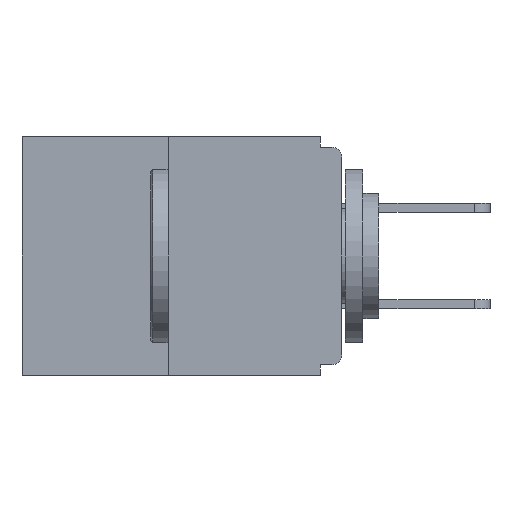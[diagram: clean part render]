
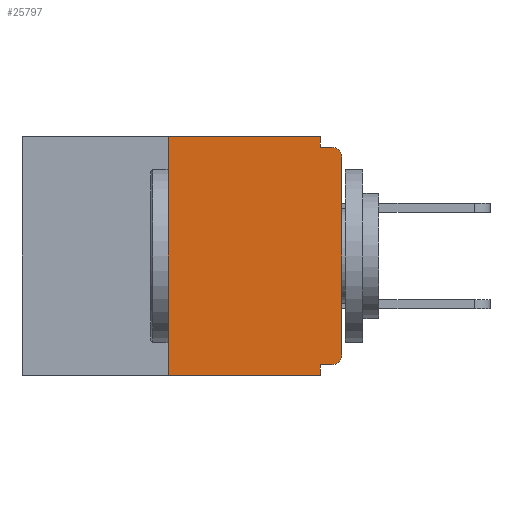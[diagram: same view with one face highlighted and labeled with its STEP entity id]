
A CAD part, left-side view. The second image highlights one B-rep face of the part: STEP entity #25797.
In plain terms, the highlighted planar face has unit normal (-1, 0, 0).
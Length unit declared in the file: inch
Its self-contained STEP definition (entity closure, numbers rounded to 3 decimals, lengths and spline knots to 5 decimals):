
#19 = VECTOR ( 'NONE', #25999, 39.37008 ) ;
#144 = DIRECTION ( 'NONE',  ( 0., -1., 0. ) ) ;
#310 = VERTEX_POINT ( 'NONE', #5713 ) ;
#333 = EDGE_CURVE ( 'NONE', #24764, #22253, #2585, .T. ) ;
#414 = DIRECTION ( 'NONE',  ( 0., -1., 0. ) ) ;
#470 = DIRECTION ( 'NONE',  ( 0., 0., -1. ) ) ;
#1014 = DIRECTION ( 'NONE',  ( 0., 0., -1. ) ) ;
#1620 = VECTOR ( 'NONE', #14173, 39.37008 ) ;
#2585 = LINE ( 'NONE', #15655, #19 ) ;
#3211 = VECTOR ( 'NONE', #24478, 39.37008 ) ;
#3716 = CARTESIAN_POINT ( 'NONE',  ( 0., 0.031, 0. ) ) ;
#3780 = EDGE_CURVE ( 'NONE', #19510, #6111, #23849, .T. ) ;
#3953 = ORIENTED_EDGE ( 'NONE', *, *, #10711, .T. ) ;
#4351 = LINE ( 'NONE', #12696, #9069 ) ;
#4534 = PLANE ( 'NONE',  #5822 ) ;
#4658 = ORIENTED_EDGE ( 'NONE', *, *, #8593, .F. ) ;
#4842 = VECTOR ( 'NONE', #414, 39.37008 ) ;
#5281 = DIRECTION ( 'NONE',  ( 0., 0., -1. ) ) ;
#5429 = ORIENTED_EDGE ( 'NONE', *, *, #17405, .F. ) ;
#5528 = CARTESIAN_POINT ( 'NONE',  ( 0., 0.25, 0. ) ) ;
#5553 = LINE ( 'NONE', #20204, #12527 ) ;
#5713 = CARTESIAN_POINT ( 'NONE',  ( 0., 0.25, -0.343 ) ) ;
#5822 = AXIS2_PLACEMENT_3D ( 'NONE', #22759, #24715, #470 ) ;
#6111 = VERTEX_POINT ( 'NONE', #15145 ) ;
#6182 = ORIENTED_EDGE ( 'NONE', *, *, #19927, .F. ) ;
#6338 = EDGE_CURVE ( 'NONE', #13359, #7127, #8822, .T. ) ;
#6804 = ORIENTED_EDGE ( 'NONE', *, *, #23769, .F. ) ;
#7127 = VERTEX_POINT ( 'NONE', #23891 ) ;
#7247 = EDGE_CURVE ( 'NONE', #21925, #22702, #4351, .T. ) ;
#7382 = DIRECTION ( 'NONE',  ( 0., 0., 1. ) ) ;
#8100 = EDGE_CURVE ( 'NONE', #6111, #13359, #17264, .T. ) ;
#8593 = EDGE_CURVE ( 'NONE', #22253, #7127, #5553, .T. ) ;
#8822 = CIRCLE ( 'NONE', #13128, 0.015 ) ;
#8937 = DIRECTION ( 'NONE',  ( -1., 0., 0. ) ) ;
#9069 = VECTOR ( 'NONE', #12786, 39.37008 ) ;
#9969 = VECTOR ( 'NONE', #21631, 39.37008 ) ;
#10627 = CARTESIAN_POINT ( 'NONE',  ( 0., 0.46, -0.343 ) ) ;
#10711 = EDGE_CURVE ( 'NONE', #310, #22702, #15845, .T. ) ;
#10890 = CARTESIAN_POINT ( 'NONE',  ( 0., 0.015, -0.03 ) ) ;
#12091 = ORIENTED_EDGE ( 'NONE', *, *, #6338, .T. ) ;
#12278 = CARTESIAN_POINT ( 'NONE',  ( 0., 0.031, -0.343 ) ) ;
#12527 = VECTOR ( 'NONE', #144, 39.37008 ) ;
#12696 = CARTESIAN_POINT ( 'NONE',  ( 0., 0.031, -0.343 ) ) ;
#12786 = DIRECTION ( 'NONE',  ( 0., 0., -1. ) ) ;
#12834 = VECTOR ( 'NONE', #7382, 39.37008 ) ;
#13128 = AXIS2_PLACEMENT_3D ( 'NONE', #10890, #8937, #1014 ) ;
#13177 = ORIENTED_EDGE ( 'NONE', *, *, #3780, .T. ) ;
#13359 = VERTEX_POINT ( 'NONE', #14010 ) ;
#13638 = EDGE_LOOP ( 'NONE', ( #6804, #6182, #3953, #22692, #5429, #13177, #14809, #12091, #4658, #19466 ) ) ;
#14010 = CARTESIAN_POINT ( 'NONE',  ( 0., 0., -0.03 ) ) ;
#14173 = DIRECTION ( 'NONE',  ( 0., 1., 0. ) ) ;
#14809 = ORIENTED_EDGE ( 'NONE', *, *, #8100, .T. ) ;
#15145 = CARTESIAN_POINT ( 'NONE',  ( 0., 0., -0.313 ) ) ;
#15655 = CARTESIAN_POINT ( 'NONE',  ( 0., 0.031, 0. ) ) ;
#15793 = LINE ( 'NONE', #26193, #1620 ) ;
#15845 = LINE ( 'NONE', #10627, #4842 ) ;
#16364 = VERTEX_POINT ( 'NONE', #25122 ) ;
#16808 = AXIS2_PLACEMENT_3D ( 'NONE', #25398, #25565, #5281 ) ;
#17264 = LINE ( 'NONE', #17635, #12834 ) ;
#17405 = EDGE_CURVE ( 'NONE', #19510, #21925, #15793, .T. ) ;
#17635 = CARTESIAN_POINT ( 'NONE',  ( 0., 0., 0. ) ) ;
#19466 = ORIENTED_EDGE ( 'NONE', *, *, #333, .F. ) ;
#19494 = FACE_OUTER_BOUND ( 'NONE', #13638, .T. ) ;
#19510 = VERTEX_POINT ( 'NONE', #20585 ) ;
#19927 = EDGE_CURVE ( 'NONE', #310, #16364, #20753, .T. ) ;
#20204 = CARTESIAN_POINT ( 'NONE',  ( 0., 0., -0.015 ) ) ;
#20550 = CARTESIAN_POINT ( 'NONE',  ( 0., 0.46, 0. ) ) ;
#20585 = CARTESIAN_POINT ( 'NONE',  ( 0., 0.015, -0.328 ) ) ;
#20753 = LINE ( 'NONE', #5528, #9969 ) ;
#21500 = LINE ( 'NONE', #20550, #3211 ) ;
#21631 = DIRECTION ( 'NONE',  ( 0., 0., 1. ) ) ;
#21925 = VERTEX_POINT ( 'NONE', #24696 ) ;
#22253 = VERTEX_POINT ( 'NONE', #25187 ) ;
#22692 = ORIENTED_EDGE ( 'NONE', *, *, #7247, .F. ) ;
#22702 = VERTEX_POINT ( 'NONE', #12278 ) ;
#22759 = CARTESIAN_POINT ( 'NONE',  ( 0., 0.46, 0. ) ) ;
#23769 = EDGE_CURVE ( 'NONE', #16364, #24764, #21500, .T. ) ;
#23849 = CIRCLE ( 'NONE', #16808, 0.015 ) ;
#23891 = CARTESIAN_POINT ( 'NONE',  ( 0., 0.015, -0.015 ) ) ;
#24478 = DIRECTION ( 'NONE',  ( 0., -1., 0. ) ) ;
#24696 = CARTESIAN_POINT ( 'NONE',  ( 0., 0.031, -0.328 ) ) ;
#24715 = DIRECTION ( 'NONE',  ( 1., 0., 0. ) ) ;
#24764 = VERTEX_POINT ( 'NONE', #3716 ) ;
#25122 = CARTESIAN_POINT ( 'NONE',  ( 0., 0.25, 0. ) ) ;
#25187 = CARTESIAN_POINT ( 'NONE',  ( 0., 0.031, -0.015 ) ) ;
#25398 = CARTESIAN_POINT ( 'NONE',  ( 0., 0.015, -0.313 ) ) ;
#25565 = DIRECTION ( 'NONE',  ( -1., 0., 0. ) ) ;
#25797 = ADVANCED_FACE ( 'NONE', ( #19494 ), #4534, .F. ) ;
#25999 = DIRECTION ( 'NONE',  ( 0., 0., -1. ) ) ;
#26193 = CARTESIAN_POINT ( 'NONE',  ( 0., 0., -0.328 ) ) ;
